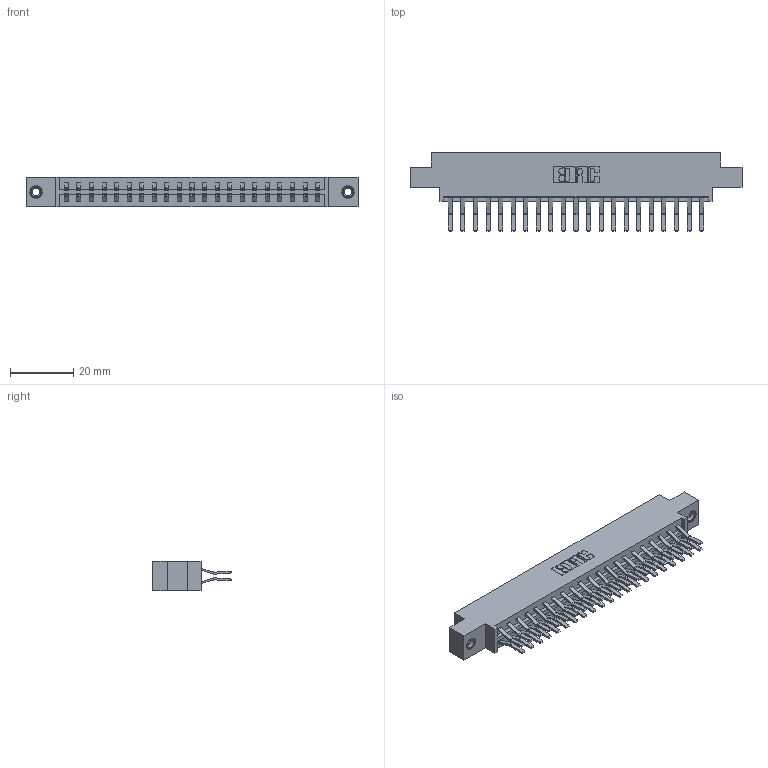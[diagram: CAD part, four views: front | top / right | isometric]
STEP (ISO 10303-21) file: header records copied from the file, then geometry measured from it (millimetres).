
FILE_DESCRIPTION (( 'STEP AP203' ), '1' );
FILE_NAME ('833-042-560-808.STEP', '2020-06-03T23:02:53', ( '' ), ( '' ), 'SwSTEP 2.0', 'SolidWorks 2020', '' );
FILE_SCHEMA (( 'CONFIG_CONTROL_DESIGN' ));
Length unit declared in the file: inch
Products named in the file (4): 833-042-560-808; 833 Part_Offset - .156 Dia - TI; 345-250-001_345-250-003-102; 345-292-001_560 Tail
Assembly tree (45 placements, depth 2):
  833-042-560-808
    833 Part_Offset - .156 Dia - TI
    345-292-001_560 Tail  x42
    345-250-001_345-250-003-102  x2
Bounding box: 104.75 x 24.78 x 9.4 mm (x, y, z)
Volume: 10538.9 mm3; surface area: 13261.9 mm2
Topology: 45 solids, 45 shells, 2446 faces, 7221 edges, 4750 vertices
Faces by surface type: plane 1618, cylinder 812, cone 12, torus 4
Entity records: 17632 total; most frequent: CARTESIAN_POINT 2933, ORIENTED_EDGE 2862, DIRECTION 2577, EDGE_CURVE 1431, VECTOR 1279, LINE 1279, VERTEX_POINT 948, AXIS2_PLACEMENT_3D 649
